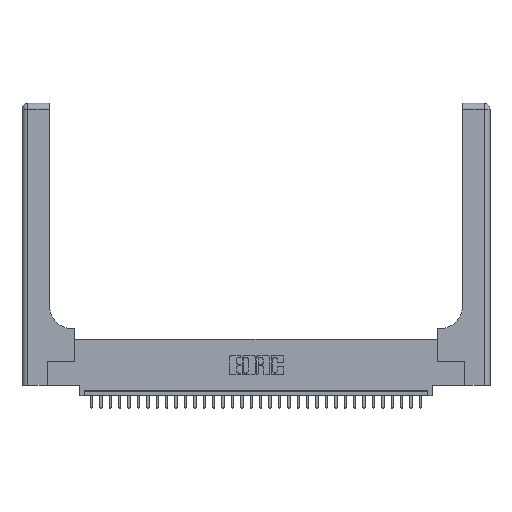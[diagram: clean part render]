
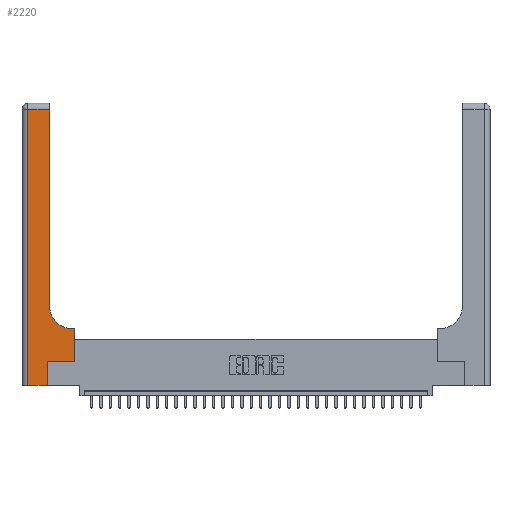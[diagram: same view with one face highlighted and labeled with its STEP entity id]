
A CAD part, top view. The second image highlights one B-rep face of the part: STEP entity #2220.
In plain terms, the highlighted planar face has unit normal (0, 0, 1).
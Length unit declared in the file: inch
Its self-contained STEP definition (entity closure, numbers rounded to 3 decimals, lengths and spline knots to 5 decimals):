
#892 = VECTOR ( 'NONE', #4041, 39.37008 ) ;
#961 = FACE_OUTER_BOUND ( 'NONE', #12026, .T. ) ;
#1662 = DIRECTION ( 'NONE',  ( -1., 0., 0. ) ) ;
#1805 = DIRECTION ( 'NONE',  ( 0., -1., 0. ) ) ;
#1973 = ORIENTED_EDGE ( 'NONE', *, *, #11355, .T. ) ;
#2111 = CARTESIAN_POINT ( 'NONE',  ( 0., 3., 0.37 ) ) ;
#2220 = ADVANCED_FACE ( 'NONE', ( #961 ), #14655, .F. ) ;
#2574 = ORIENTED_EDGE ( 'NONE', *, *, #18387, .T. ) ;
#3121 = DIRECTION ( 'NONE',  ( 1., 0., 0. ) ) ;
#3123 = LINE ( 'NONE', #22144, #9616 ) ;
#3380 = DIRECTION ( 'NONE',  ( 0., 1., 0. ) ) ;
#3432 = CARTESIAN_POINT ( 'NONE',  ( 0.269, 0., 0.37 ) ) ;
#3575 = EDGE_CURVE ( 'NONE', #20229, #25351, #16190, .T. ) ;
#3580 = EDGE_CURVE ( 'NONE', #19134, #4356, #27350, .T. ) ;
#4041 = DIRECTION ( 'NONE',  ( 0., 1., 0. ) ) ;
#4356 = VERTEX_POINT ( 'NONE', #8476 ) ;
#4814 = VECTOR ( 'NONE', #3121, 39.37008 ) ;
#5187 = CIRCLE ( 'NONE', #15766, 0.25 ) ;
#5404 = ORIENTED_EDGE ( 'NONE', *, *, #11868, .T. ) ;
#6029 = VERTEX_POINT ( 'NONE', #23811 ) ;
#6434 = CARTESIAN_POINT ( 'NONE',  ( 0.269, 0., 0.37 ) ) ;
#6539 = ORIENTED_EDGE ( 'NONE', *, *, #18289, .T. ) ;
#7357 = ORIENTED_EDGE ( 'NONE', *, *, #3580, .T. ) ;
#7623 = DIRECTION ( 'NONE',  ( 1., 0., 0. ) ) ;
#8476 = CARTESIAN_POINT ( 'NONE',  ( 0.06, 2.94, 0.37 ) ) ;
#8794 = AXIS2_PLACEMENT_3D ( 'NONE', #2111, #20085, #31249 ) ;
#8808 = VERTEX_POINT ( 'NONE', #24993 ) ;
#9616 = VECTOR ( 'NONE', #1805, 39.37008 ) ;
#9989 = VECTOR ( 'NONE', #3380, 39.37008 ) ;
#10071 = DIRECTION ( 'NONE',  ( 1., 0., 0. ) ) ;
#11187 = CARTESIAN_POINT ( 'NONE',  ( 0.5585, 0.25, 0.37 ) ) ;
#11355 = EDGE_CURVE ( 'NONE', #8808, #19134, #12783, .T. ) ;
#11732 = CARTESIAN_POINT ( 'NONE',  ( 0.269, 0.25, 0.37 ) ) ;
#11868 = EDGE_CURVE ( 'NONE', #4356, #26101, #3123, .T. ) ;
#12026 = EDGE_LOOP ( 'NONE', ( #1973, #7357, #5404, #23249, #2574, #25490, #20739, #13335, #6539 ) ) ;
#12299 = DIRECTION ( 'NONE',  ( 0., 1., 0. ) ) ;
#12731 = CARTESIAN_POINT ( 'NONE',  ( 0.269, 0.25, 0.37 ) ) ;
#12783 = LINE ( 'NONE', #16130, #9989 ) ;
#12871 = DIRECTION ( 'NONE',  ( 0., 0., -1. ) ) ;
#12926 = CARTESIAN_POINT ( 'NONE',  ( 0., 0., 0.37 ) ) ;
#13335 = ORIENTED_EDGE ( 'NONE', *, *, #24884, .T. ) ;
#13772 = VECTOR ( 'NONE', #24923, 39.37008 ) ;
#14655 = PLANE ( 'NONE',  #8794 ) ;
#15729 = CARTESIAN_POINT ( 'NONE',  ( 0.5585, 0.6, 0.37 ) ) ;
#15766 = AXIS2_PLACEMENT_3D ( 'NONE', #29901, #12871, #10071 ) ;
#16049 = CARTESIAN_POINT ( 'NONE',  ( 0.06, 0., 0.37 ) ) ;
#16130 = CARTESIAN_POINT ( 'NONE',  ( 0.2915, 3., 0.37 ) ) ;
#16190 = LINE ( 'NONE', #16600, #26550 ) ;
#16600 = CARTESIAN_POINT ( 'NONE',  ( 0.5585, 0.25, 0.37 ) ) ;
#17253 = EDGE_CURVE ( 'NONE', #30557, #20229, #29654, .T. ) ;
#18289 = EDGE_CURVE ( 'NONE', #6029, #8808, #5187, .T. ) ;
#18387 = EDGE_CURVE ( 'NONE', #25434, #30557, #33007, .T. ) ;
#19134 = VERTEX_POINT ( 'NONE', #28676 ) ;
#20085 = DIRECTION ( 'NONE',  ( 0., 0., -1. ) ) ;
#20229 = VERTEX_POINT ( 'NONE', #11187 ) ;
#20565 = EDGE_CURVE ( 'NONE', #26101, #25434, #22420, .T. ) ;
#20628 = LINE ( 'NONE', #32962, #21866 ) ;
#20739 = ORIENTED_EDGE ( 'NONE', *, *, #3575, .T. ) ;
#21866 = VECTOR ( 'NONE', #1662, 39.37008 ) ;
#22144 = CARTESIAN_POINT ( 'NONE',  ( 0.06, 3., 0.37 ) ) ;
#22420 = LINE ( 'NONE', #12926, #25228 ) ;
#23249 = ORIENTED_EDGE ( 'NONE', *, *, #20565, .T. ) ;
#23811 = CARTESIAN_POINT ( 'NONE',  ( 0.5415, 0.6, 0.37 ) ) ;
#24884 = EDGE_CURVE ( 'NONE', #25351, #6029, #20628, .T. ) ;
#24923 = DIRECTION ( 'NONE',  ( -1., 0., 0. ) ) ;
#24993 = CARTESIAN_POINT ( 'NONE',  ( 0.2915, 0.85, 0.37 ) ) ;
#25228 = VECTOR ( 'NONE', #7623, 39.37008 ) ;
#25351 = VERTEX_POINT ( 'NONE', #15729 ) ;
#25434 = VERTEX_POINT ( 'NONE', #3432 ) ;
#25490 = ORIENTED_EDGE ( 'NONE', *, *, #17253, .T. ) ;
#26101 = VERTEX_POINT ( 'NONE', #16049 ) ;
#26550 = VECTOR ( 'NONE', #12299, 39.37008 ) ;
#27350 = LINE ( 'NONE', #30512, #13772 ) ;
#28676 = CARTESIAN_POINT ( 'NONE',  ( 0.2915, 2.94, 0.37 ) ) ;
#29654 = LINE ( 'NONE', #12731, #4814 ) ;
#29901 = CARTESIAN_POINT ( 'NONE',  ( 0.5415, 0.85, 0.37 ) ) ;
#30512 = CARTESIAN_POINT ( 'NONE',  ( 0., 2.94, 0.37 ) ) ;
#30557 = VERTEX_POINT ( 'NONE', #11732 ) ;
#31249 = DIRECTION ( 'NONE',  ( -1., 0., 0. ) ) ;
#32962 = CARTESIAN_POINT ( 'NONE',  ( 0.2915, 0.6, 0.37 ) ) ;
#33007 = LINE ( 'NONE', #6434, #892 ) ;
